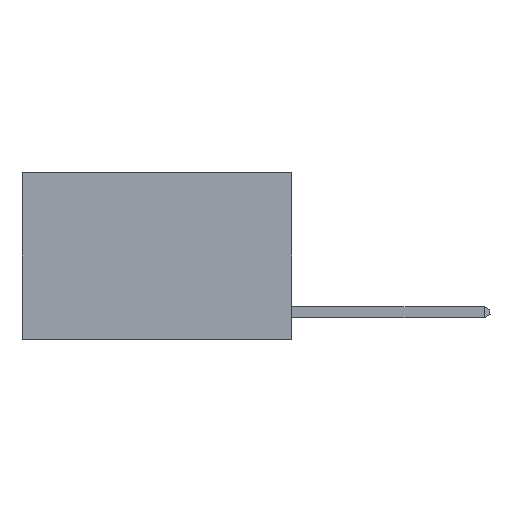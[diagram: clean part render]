
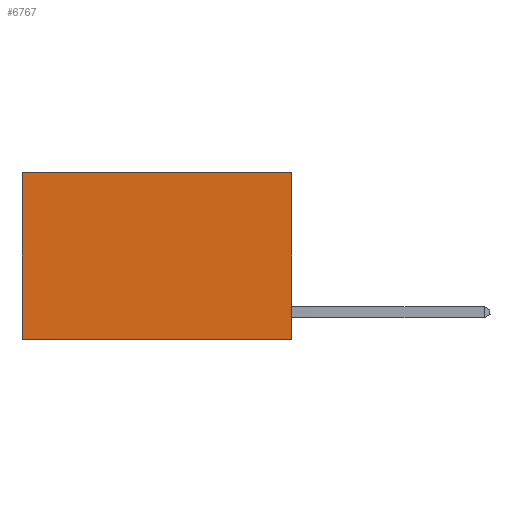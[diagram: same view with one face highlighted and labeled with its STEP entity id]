
A CAD part, left-side view. The second image highlights one B-rep face of the part: STEP entity #6767.
In plain terms, the highlighted planar face has unit normal (-1, 0, 0).
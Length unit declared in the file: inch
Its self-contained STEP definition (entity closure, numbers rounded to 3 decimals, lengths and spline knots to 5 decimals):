
#180 = CARTESIAN_POINT ( 'NONE',  ( 0.2625, 0.6, -0.37 ) ) ;
#382 = VECTOR ( 'NONE', #4091, 39.37008 ) ;
#2153 = CARTESIAN_POINT ( 'NONE',  ( 0.2625, 0., -0.37 ) ) ;
#2335 = DIRECTION ( 'NONE',  ( 0., 0., -1. ) ) ;
#2825 = DIRECTION ( 'NONE',  ( 0., 1., 0. ) ) ;
#3005 = EDGE_CURVE ( 'NONE', #7701, #7827, #13242, .T. ) ;
#3025 = ORIENTED_EDGE ( 'NONE', *, *, #3005, .T. ) ;
#3187 = CARTESIAN_POINT ( 'NONE',  ( 0.2625, 0., 0. ) ) ;
#3557 = EDGE_CURVE ( 'NONE', #7827, #4080, #7921, .T. ) ;
#4080 = VERTEX_POINT ( 'NONE', #180 ) ;
#4091 = DIRECTION ( 'NONE',  ( 0., 1., 0. ) ) ;
#4230 = EDGE_CURVE ( 'NONE', #7701, #10872, #5585, .T. ) ;
#4457 = VECTOR ( 'NONE', #2825, 39.37008 ) ;
#4939 = VECTOR ( 'NONE', #2335, 39.37008 ) ;
#5585 = LINE ( 'NONE', #10235, #12772 ) ;
#6015 = ORIENTED_EDGE ( 'NONE', *, *, #3557, .T. ) ;
#6139 = CARTESIAN_POINT ( 'NONE',  ( 0.2625, 0., -0.37 ) ) ;
#6446 = PLANE ( 'NONE',  #12067 ) ;
#6767 = ADVANCED_FACE ( 'NONE', ( #12519 ), #6446, .F. ) ;
#7395 = CARTESIAN_POINT ( 'NONE',  ( 0.2625, 0., 0. ) ) ;
#7701 = VERTEX_POINT ( 'NONE', #3187 ) ;
#7827 = VERTEX_POINT ( 'NONE', #12867 ) ;
#7921 = LINE ( 'NONE', #11528, #4939 ) ;
#8809 = LINE ( 'NONE', #6139, #382 ) ;
#8815 = DIRECTION ( 'NONE',  ( 1., 0., 0. ) ) ;
#8966 = DIRECTION ( 'NONE',  ( 0., 0., -1. ) ) ;
#9437 = EDGE_CURVE ( 'NONE', #10872, #4080, #8809, .T. ) ;
#10235 = CARTESIAN_POINT ( 'NONE',  ( 0.2625, 0., 0. ) ) ;
#10872 = VERTEX_POINT ( 'NONE', #2153 ) ;
#11528 = CARTESIAN_POINT ( 'NONE',  ( 0.2625, 0.6, 0. ) ) ;
#12067 = AXIS2_PLACEMENT_3D ( 'NONE', #14656, #8815, #8966 ) ;
#12519 = FACE_OUTER_BOUND ( 'NONE', #14710, .T. ) ;
#12772 = VECTOR ( 'NONE', #13636, 39.37008 ) ;
#12867 = CARTESIAN_POINT ( 'NONE',  ( 0.2625, 0.6, 0. ) ) ;
#13038 = ORIENTED_EDGE ( 'NONE', *, *, #9437, .F. ) ;
#13242 = LINE ( 'NONE', #7395, #4457 ) ;
#13276 = ORIENTED_EDGE ( 'NONE', *, *, #4230, .F. ) ;
#13636 = DIRECTION ( 'NONE',  ( 0., 0., -1. ) ) ;
#14656 = CARTESIAN_POINT ( 'NONE',  ( 0.2625, 0., 0. ) ) ;
#14710 = EDGE_LOOP ( 'NONE', ( #6015, #13038, #13276, #3025 ) ) ;
